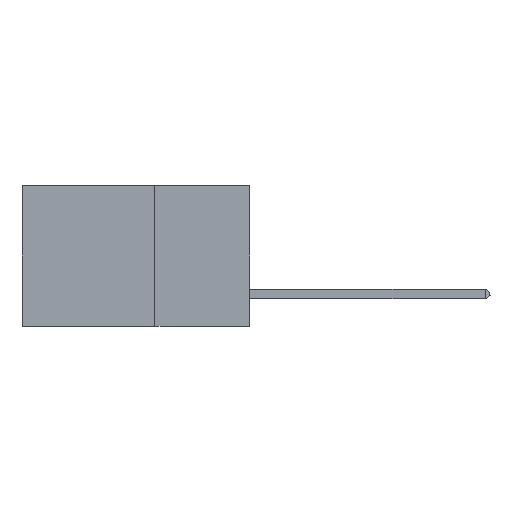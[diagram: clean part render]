
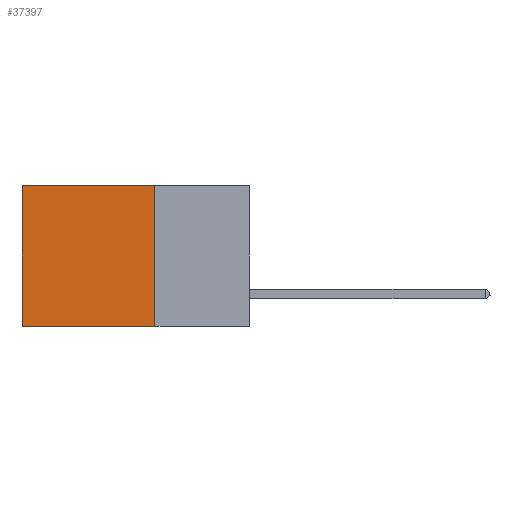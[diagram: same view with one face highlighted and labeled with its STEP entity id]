
A CAD part, left-side view. The second image highlights one B-rep face of the part: STEP entity #37397.
In plain terms, the highlighted planar face has unit normal (-1, 0, 0).
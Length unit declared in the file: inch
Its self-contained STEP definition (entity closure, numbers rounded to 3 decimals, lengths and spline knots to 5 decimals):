
#946 = AXIS2_PLACEMENT_3D ( 'NONE', #19604, #13034, #19209 ) ;
#1024 = FACE_OUTER_BOUND ( 'NONE', #7544, .T. ) ;
#1667 = VECTOR ( 'NONE', #19241, 39.37008 ) ;
#1705 = EDGE_CURVE ( 'NONE', #12413, #9142, #8331, .T. ) ;
#1841 = VERTEX_POINT ( 'NONE', #19266 ) ;
#2707 = CARTESIAN_POINT ( 'NONE',  ( 0.2875, 0.25, 0. ) ) ;
#3535 = VECTOR ( 'NONE', #30062, 39.37008 ) ;
#4618 = CARTESIAN_POINT ( 'NONE',  ( 0.2875, 0.6, 0. ) ) ;
#7544 = EDGE_LOOP ( 'NONE', ( #16542, #25519, #29143, #27809 ) ) ;
#8331 = LINE ( 'NONE', #33091, #15696 ) ;
#8700 = VECTOR ( 'NONE', #13965, 39.37008 ) ;
#9142 = VERTEX_POINT ( 'NONE', #37892 ) ;
#12413 = VERTEX_POINT ( 'NONE', #4618 ) ;
#13034 = DIRECTION ( 'NONE',  ( 1., 0., 0. ) ) ;
#13610 = PLANE ( 'NONE',  #946 ) ;
#13965 = DIRECTION ( 'NONE',  ( 0., 1., 0. ) ) ;
#14573 = LINE ( 'NONE', #32711, #8700 ) ;
#15696 = VECTOR ( 'NONE', #17917, 39.37008 ) ;
#16542 = ORIENTED_EDGE ( 'NONE', *, *, #1705, .T. ) ;
#16768 = CARTESIAN_POINT ( 'NONE',  ( 0.2875, 0.25, 0. ) ) ;
#17917 = DIRECTION ( 'NONE',  ( 0., 0., -1. ) ) ;
#18061 = VERTEX_POINT ( 'NONE', #16768 ) ;
#19209 = DIRECTION ( 'NONE',  ( 0., 0., -1. ) ) ;
#19241 = DIRECTION ( 'NONE',  ( 0., 1., 0. ) ) ;
#19266 = CARTESIAN_POINT ( 'NONE',  ( 0.2875, 0.25, -0.37 ) ) ;
#19604 = CARTESIAN_POINT ( 'NONE',  ( 0.2875, 0.25, 0. ) ) ;
#19646 = LINE ( 'NONE', #37602, #1667 ) ;
#24599 = EDGE_CURVE ( 'NONE', #18061, #12413, #14573, .T. ) ;
#24854 = EDGE_CURVE ( 'NONE', #1841, #9142, #19646, .T. ) ;
#25519 = ORIENTED_EDGE ( 'NONE', *, *, #24854, .F. ) ;
#27809 = ORIENTED_EDGE ( 'NONE', *, *, #24599, .T. ) ;
#29143 = ORIENTED_EDGE ( 'NONE', *, *, #36041, .F. ) ;
#30062 = DIRECTION ( 'NONE',  ( 0., 0., -1. ) ) ;
#32711 = CARTESIAN_POINT ( 'NONE',  ( 0.2875, 0.25, 0. ) ) ;
#33091 = CARTESIAN_POINT ( 'NONE',  ( 0.2875, 0.6, 0. ) ) ;
#36041 = EDGE_CURVE ( 'NONE', #18061, #1841, #39235, .T. ) ;
#37397 = ADVANCED_FACE ( 'NONE', ( #1024 ), #13610, .F. ) ;
#37602 = CARTESIAN_POINT ( 'NONE',  ( 0.2875, 0.25, -0.37 ) ) ;
#37892 = CARTESIAN_POINT ( 'NONE',  ( 0.2875, 0.6, -0.37 ) ) ;
#39235 = LINE ( 'NONE', #2707, #3535 ) ;
